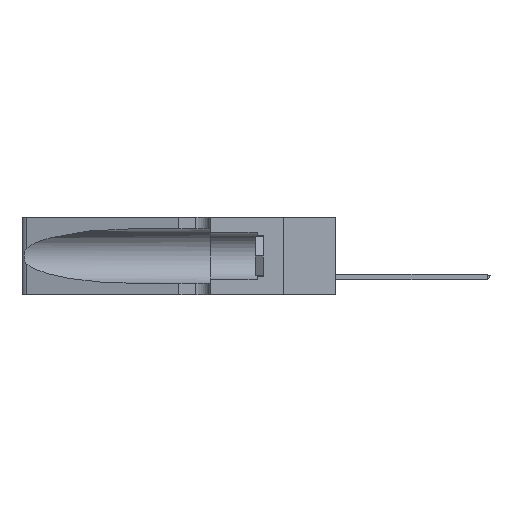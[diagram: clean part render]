
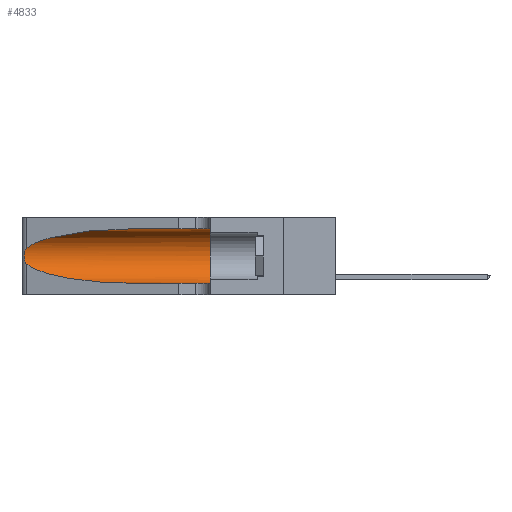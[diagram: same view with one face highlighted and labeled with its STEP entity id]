
A CAD part, left-side view. The second image highlights one B-rep face of the part: STEP entity #4833.
In plain terms, the highlighted cylindrical face has radius 3.308 mm (diameter 6.617 mm), a partial arc.
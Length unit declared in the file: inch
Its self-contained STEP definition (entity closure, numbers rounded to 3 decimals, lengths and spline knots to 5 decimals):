
#163 = EDGE_CURVE ( 'NONE', #15642, #28654, #30024, .T. ) ;
#260 = CARTESIAN_POINT ( 'NONE',  ( 0.25487, 1.22718, 0.22369 ) ) ;
#612 = CARTESIAN_POINT ( 'NONE',  ( 0.18966, 0.96281, 0.05475 ) ) ;
#2104 = CARTESIAN_POINT ( 'NONE',  ( 0.25555, 1.22993, 0.14849 ) ) ;
#4105 = EDGE_CURVE ( 'NONE', #14425, #47035, #22413, .T. ) ;
#4202 = CARTESIAN_POINT ( 'NONE',  ( 0.1305, 0.35, 0.31525 ) ) ;
#4227 = DIRECTION ( 'NONE',  ( 0., -1., 0. ) ) ;
#4763 = CARTESIAN_POINT ( 'NONE',  ( 0.1305, 0.72297, 0.05475 ) ) ;
#4833 = ADVANCED_FACE ( 'NONE', ( #51203 ), #39241, .F. ) ;
#5220 = DIRECTION ( 'NONE',  ( 0., 1., 0. ) ) ;
#5292 = CARTESIAN_POINT ( 'NONE',  ( 0.25487, 1.22718, 0.14631 ) ) ;
#5750 = CARTESIAN_POINT ( 'NONE',  ( 0.1305, 0.35, 0.185 ) ) ;
#5889 = CARTESIAN_POINT ( 'NONE',  ( 0.1305, 0.35, 0.05475 ) ) ;
#7300 = CARTESIAN_POINT ( 'NONE',  ( 0.25787, 1.23484, 0.2124 ) ) ;
#7913 = DIRECTION ( 'NONE',  ( 0., 0., -1. ) ) ;
#9061 = VECTOR ( 'NONE', #9472, 39.37008 ) ;
#9440 = EDGE_CURVE ( 'NONE', #51798, #14425, #39462, .T. ) ;
#9472 = DIRECTION ( 'NONE',  ( 0., -1., 0. ) ) ;
#10564 = CARTESIAN_POINT ( 'NONE',  ( 0.1305, 1.61858, 0.05475 ) ) ;
#11785 = VERTEX_POINT ( 'NONE', #4202 ) ;
#11897 = CARTESIAN_POINT ( 'NONE',  ( 0.26018, 1.23835, 0.19895 ) ) ;
#12561 = CARTESIAN_POINT ( 'NONE',  ( 0.25789, 1.23486, 0.15765 ) ) ;
#13488 = ORIENTED_EDGE ( 'NONE', *, *, #29544, .F. ) ;
#14425 = VERTEX_POINT ( 'NONE', #41225 ) ;
#14453 = CIRCLE ( 'NONE', #20141, 0.13025 ) ;
#15062 = CARTESIAN_POINT ( 'NONE',  ( 0.25555, 1.22994, 0.2215 ) ) ;
#15642 = VERTEX_POINT ( 'NONE', #37574 ) ;
#15884 = CARTESIAN_POINT ( 'NONE',  ( 0.1305, 1.61858, 0.185 ) ) ;
#16694 = ORIENTED_EDGE ( 'NONE', *, *, #163, .T. ) ;
#17398 = DIRECTION ( 'NONE',  ( 0., 0., 1. ) ) ;
#19089 = ORIENTED_EDGE ( 'NONE', *, *, #45110, .T. ) ;
#19465 = LINE ( 'NONE', #20355, #33933 ) ;
#19672 = CARTESIAN_POINT ( 'NONE',  ( 0.25854, 1.2359, 0.20912 ) ) ;
#20141 = AXIS2_PLACEMENT_3D ( 'NONE', #5750, #5220, #17398 ) ;
#20355 = CARTESIAN_POINT ( 'NONE',  ( 0.1305, 1.61858, 0.31525 ) ) ;
#20754 = CARTESIAN_POINT ( 'NONE',  ( 0.25487, 1.22718, 0.22369 ) ) ;
#21814 = ORIENTED_EDGE ( 'NONE', *, *, #9440, .T. ) ;
#22369 = CARTESIAN_POINT ( 'NONE',  ( 0.25639, 1.23186, 0.15144 ) ) ;
#22413 = LINE ( 'NONE', #10564, #9061 ) ;
#23326 = AXIS2_PLACEMENT_3D ( 'NONE', #15884, #48169, #7913 ) ;
#25415 = CARTESIAN_POINT ( 'NONE',  ( 0.26017, 1.23833, 0.17102 ) ) ;
#27587 = CARTESIAN_POINT ( 'NONE',  ( 0.25639, 1.23184, 0.21858 ) ) ;
#28654 = VERTEX_POINT ( 'NONE', #20754 ) ;
#29538 = EDGE_LOOP ( 'NONE', ( #16694, #19089, #21814, #40222, #13488, #48259 ) ) ;
#29544 = EDGE_CURVE ( 'NONE', #11785, #47035, #14453, .T. ) ;
#30024 =( BOUNDED_CURVE ( )  B_SPLINE_CURVE ( 3, ( #36888, #45195, #33139, #260 ),
 .UNSPECIFIED., .F., .T. ) 
 B_SPLINE_CURVE_WITH_KNOTS ( ( 4, 4 ),
 ( 1.5708, 2.84003 ),
 .UNSPECIFIED. ) 
 CURVE ( )  GEOMETRIC_REPRESENTATION_ITEM ( )  RATIONAL_B_SPLINE_CURVE ( ( 1., 0.87, 0.87, 1. ) ) 
 REPRESENTATION_ITEM ( '' )  );
#31408 = CARTESIAN_POINT ( 'NONE',  ( 0.25487, 1.22718, 0.14631 ) ) ;
#32278 = CARTESIAN_POINT ( 'NONE',  ( 0.26075, 1.23896, 0.19203 ) ) ;
#33139 = CARTESIAN_POINT ( 'NONE',  ( 0.2373, 1.15595, 0.28018 ) ) ;
#33933 = VECTOR ( 'NONE', #4227, 39.37008 ) ;
#35618 = B_SPLINE_CURVE_WITH_KNOTS ( 'NONE', 3,
 ( #39447, #15062, #27587, #7300, #19672, #11897, #32278, #51842, #25415, #42377, #12561, #22369, #2104, #31408 ),
 .UNSPECIFIED., .F., .F.,
 ( 4, 2, 2, 2, 2, 2, 4 ),
 ( 0., 0.00027, 0.00053, 0.00107, 0.0016, 0.00187, 0.00214 ),
 .UNSPECIFIED. ) ;
#36888 = CARTESIAN_POINT ( 'NONE',  ( 0.1305, 0.72297, 0.31525 ) ) ;
#37574 = CARTESIAN_POINT ( 'NONE',  ( 0.1305, 0.72297, 0.31525 ) ) ;
#39241 = CYLINDRICAL_SURFACE ( 'NONE', #23326, 0.13025 ) ;
#39447 = CARTESIAN_POINT ( 'NONE',  ( 0.25487, 1.22718, 0.22369 ) ) ;
#39462 =( BOUNDED_CURVE ( )  B_SPLINE_CURVE ( 3, ( #5292, #49935, #612, #4763 ),
 .UNSPECIFIED., .F., .T. ) 
 B_SPLINE_CURVE_WITH_KNOTS ( ( 4, 4 ),
 ( 3.44316, 4.71239 ),
 .UNSPECIFIED. ) 
 CURVE ( )  GEOMETRIC_REPRESENTATION_ITEM ( )  RATIONAL_B_SPLINE_CURVE ( ( 1., 0.87, 0.87, 1. ) ) 
 REPRESENTATION_ITEM ( '' )  );
#40170 = EDGE_CURVE ( 'NONE', #15642, #11785, #19465, .T. ) ;
#40222 = ORIENTED_EDGE ( 'NONE', *, *, #4105, .T. ) ;
#41225 = CARTESIAN_POINT ( 'NONE',  ( 0.1305, 0.72297, 0.05475 ) ) ;
#42377 = CARTESIAN_POINT ( 'NONE',  ( 0.25856, 1.23593, 0.16098 ) ) ;
#45110 = EDGE_CURVE ( 'NONE', #28654, #51798, #35618, .T. ) ;
#45195 = CARTESIAN_POINT ( 'NONE',  ( 0.18966, 0.96281, 0.31525 ) ) ;
#47035 = VERTEX_POINT ( 'NONE', #5889 ) ;
#48169 = DIRECTION ( 'NONE',  ( 0., -1., 0. ) ) ;
#48259 = ORIENTED_EDGE ( 'NONE', *, *, #40170, .F. ) ;
#49692 = CARTESIAN_POINT ( 'NONE',  ( 0.25487, 1.22718, 0.14631 ) ) ;
#49935 = CARTESIAN_POINT ( 'NONE',  ( 0.2373, 1.15595, 0.08982 ) ) ;
#51203 = FACE_OUTER_BOUND ( 'NONE', #29538, .T. ) ;
#51798 = VERTEX_POINT ( 'NONE', #49692 ) ;
#51842 = CARTESIAN_POINT ( 'NONE',  ( 0.26075, 1.23896, 0.178 ) ) ;
